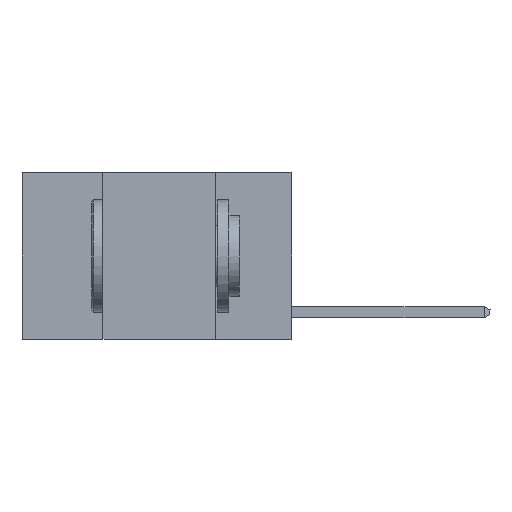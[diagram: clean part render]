
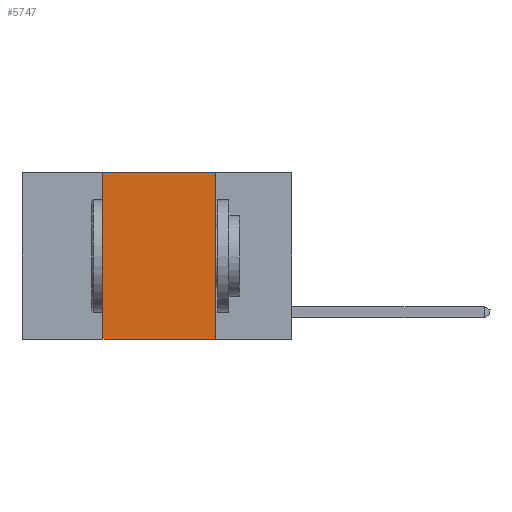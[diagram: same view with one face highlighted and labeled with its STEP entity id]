
A CAD part, left-side view. The second image highlights one B-rep face of the part: STEP entity #5747.
In plain terms, the highlighted planar face has unit normal (-1, 0, 0).
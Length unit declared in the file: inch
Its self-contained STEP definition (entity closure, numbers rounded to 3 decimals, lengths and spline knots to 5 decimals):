
#1201 = CARTESIAN_POINT ( 'NONE',  ( 0., 0.42, 0. ) ) ;
#1574 = ORIENTED_EDGE ( 'NONE', *, *, #7519, .F. ) ;
#1892 = VECTOR ( 'NONE', #8014, 39.37008 ) ;
#3248 = LINE ( 'NONE', #9055, #16750 ) ;
#3324 = FACE_OUTER_BOUND ( 'NONE', #16250, .T. ) ;
#4332 = VERTEX_POINT ( 'NONE', #12542 ) ;
#4799 = CARTESIAN_POINT ( 'NONE',  ( 0., 0.6, 0. ) ) ;
#4889 = PLANE ( 'NONE',  #13885 ) ;
#5345 = LINE ( 'NONE', #15345, #7117 ) ;
#5747 = ADVANCED_FACE ( 'NONE', ( #3324 ), #4889, .F. ) ;
#6114 = DIRECTION ( 'NONE',  ( 1., 0., 0. ) ) ;
#6130 = VECTOR ( 'NONE', #10699, 39.37008 ) ;
#6206 = CARTESIAN_POINT ( 'NONE',  ( 0., 0.42, -0.37 ) ) ;
#6368 = ORIENTED_EDGE ( 'NONE', *, *, #16730, .F. ) ;
#7117 = VECTOR ( 'NONE', #8184, 39.37008 ) ;
#7519 = EDGE_CURVE ( 'NONE', #7677, #14432, #9202, .T. ) ;
#7677 = VERTEX_POINT ( 'NONE', #9591 ) ;
#8014 = DIRECTION ( 'NONE',  ( 0., 0., 1. ) ) ;
#8184 = DIRECTION ( 'NONE',  ( 0., -1., 0. ) ) ;
#8937 = DIRECTION ( 'NONE',  ( 0., 0., -1. ) ) ;
#9055 = CARTESIAN_POINT ( 'NONE',  ( 0., 0.17, 0. ) ) ;
#9105 = CARTESIAN_POINT ( 'NONE',  ( 0., 0.6, 0. ) ) ;
#9147 = VERTEX_POINT ( 'NONE', #6206 ) ;
#9202 = LINE ( 'NONE', #9105, #6130 ) ;
#9591 = CARTESIAN_POINT ( 'NONE',  ( 0., 0.42, 0. ) ) ;
#10699 = DIRECTION ( 'NONE',  ( 0., -1., 0. ) ) ;
#10937 = CARTESIAN_POINT ( 'NONE',  ( 0., 0.17, 0. ) ) ;
#11501 = ORIENTED_EDGE ( 'NONE', *, *, #17057, .T. ) ;
#12542 = CARTESIAN_POINT ( 'NONE',  ( 0., 0.17, -0.37 ) ) ;
#13885 = AXIS2_PLACEMENT_3D ( 'NONE', #4799, #6114, #8937 ) ;
#14432 = VERTEX_POINT ( 'NONE', #10937 ) ;
#14783 = DIRECTION ( 'NONE',  ( 0., 0., -1. ) ) ;
#15345 = CARTESIAN_POINT ( 'NONE',  ( 0., 0.6, -0.37 ) ) ;
#16250 = EDGE_LOOP ( 'NONE', ( #17442, #1574, #6368, #11501 ) ) ;
#16606 = LINE ( 'NONE', #1201, #1892 ) ;
#16730 = EDGE_CURVE ( 'NONE', #9147, #7677, #16606, .T. ) ;
#16750 = VECTOR ( 'NONE', #14783, 39.37008 ) ;
#17057 = EDGE_CURVE ( 'NONE', #9147, #4332, #5345, .T. ) ;
#17442 = ORIENTED_EDGE ( 'NONE', *, *, #17869, .F. ) ;
#17869 = EDGE_CURVE ( 'NONE', #14432, #4332, #3248, .T. ) ;
